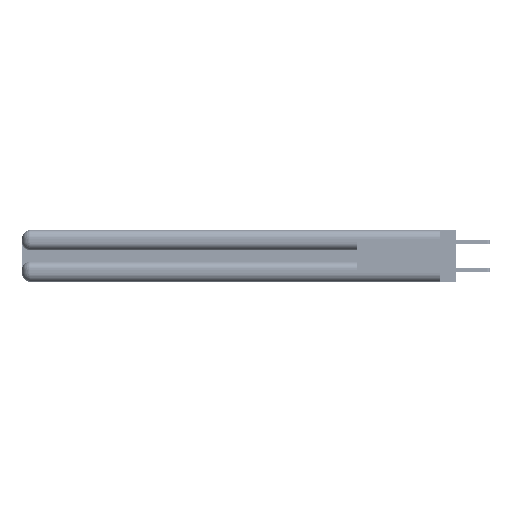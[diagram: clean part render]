
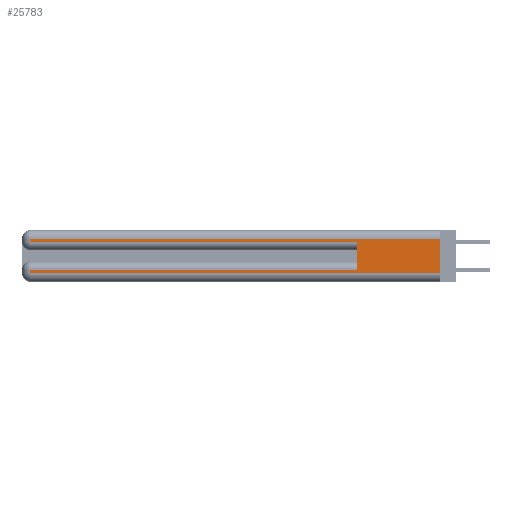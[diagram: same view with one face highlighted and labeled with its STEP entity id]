
A CAD part, left-side view. The second image highlights one B-rep face of the part: STEP entity #25783.
In plain terms, the highlighted planar face has unit normal (-1, 0, 0).
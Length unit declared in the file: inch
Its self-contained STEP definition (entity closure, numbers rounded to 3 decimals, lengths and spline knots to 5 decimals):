
#745 = EDGE_CURVE ( 'NONE', #26347, #50135, #25596, .T. ) ;
#1345 = CARTESIAN_POINT ( 'NONE',  ( 0., 0., 0.085 ) ) ;
#2168 = VERTEX_POINT ( 'NONE', #16665 ) ;
#4314 = CARTESIAN_POINT ( 'NONE',  ( 0., 2.94, 0.31 ) ) ;
#6376 = VERTEX_POINT ( 'NONE', #28918 ) ;
#7608 = PLANE ( 'NONE',  #21786 ) ;
#8194 = EDGE_CURVE ( 'NONE', #26347, #46126, #44159, .T. ) ;
#8796 = CARTESIAN_POINT ( 'NONE',  ( 0., 0.6, 0.285 ) ) ;
#9273 = ORIENTED_EDGE ( 'NONE', *, *, #20808, .T. ) ;
#9450 = ORIENTED_EDGE ( 'NONE', *, *, #745, .F. ) ;
#10535 = LINE ( 'NONE', #53746, #53653 ) ;
#10716 = LINE ( 'NONE', #10890, #23143 ) ;
#10890 = CARTESIAN_POINT ( 'NONE',  ( 0., 0., 0.285 ) ) ;
#10915 = CARTESIAN_POINT ( 'NONE',  ( 0., 0., 0.06 ) ) ;
#11662 = DIRECTION ( 'NONE',  ( 0., 0., 1. ) ) ;
#14680 = VECTOR ( 'NONE', #11662, 39.37008 ) ;
#14950 = VECTOR ( 'NONE', #29302, 39.37008 ) ;
#15764 = DIRECTION ( 'NONE',  ( 0., -1., 0. ) ) ;
#16665 = CARTESIAN_POINT ( 'NONE',  ( 0., 2.94, 0.06 ) ) ;
#16759 = EDGE_CURVE ( 'NONE', #42700, #2168, #10535, .T. ) ;
#19677 = CARTESIAN_POINT ( 'NONE',  ( 0., 2.94, 0.37 ) ) ;
#20808 = EDGE_CURVE ( 'NONE', #2168, #50135, #25682, .T. ) ;
#21786 = AXIS2_PLACEMENT_3D ( 'NONE', #25414, #38299, #34571 ) ;
#23143 = VECTOR ( 'NONE', #41982, 39.37008 ) ;
#23266 = EDGE_LOOP ( 'NONE', ( #9450, #26872, #36461, #52309, #53815, #45642, #42900, #9273 ) ) ;
#24949 = VECTOR ( 'NONE', #15764, 39.37008 ) ;
#25392 = VECTOR ( 'NONE', #55102, 39.37008 ) ;
#25414 = CARTESIAN_POINT ( 'NONE',  ( 0., 0., 0.37 ) ) ;
#25596 = LINE ( 'NONE', #37191, #54187 ) ;
#25682 = LINE ( 'NONE', #10915, #24949 ) ;
#25783 = ADVANCED_FACE ( 'NONE', ( #51141 ), #7608, .F. ) ;
#26238 = EDGE_CURVE ( 'NONE', #49688, #30802, #10716, .T. ) ;
#26347 = VERTEX_POINT ( 'NONE', #55228 ) ;
#26872 = ORIENTED_EDGE ( 'NONE', *, *, #8194, .T. ) ;
#28918 = CARTESIAN_POINT ( 'NONE',  ( 0., 0.6, 0.085 ) ) ;
#29302 = DIRECTION ( 'NONE',  ( 0., 1., 0. ) ) ;
#30802 = VERTEX_POINT ( 'NONE', #8796 ) ;
#33212 = CARTESIAN_POINT ( 'NONE',  ( 0., 0., 0.31 ) ) ;
#34571 = DIRECTION ( 'NONE',  ( 0., 0., -1. ) ) ;
#35646 = EDGE_CURVE ( 'NONE', #6376, #30802, #49414, .T. ) ;
#36461 = ORIENTED_EDGE ( 'NONE', *, *, #36992, .T. ) ;
#36992 = EDGE_CURVE ( 'NONE', #46126, #49688, #57228, .T. ) ;
#37191 = CARTESIAN_POINT ( 'NONE',  ( 0., 0., 0.37 ) ) ;
#38299 = DIRECTION ( 'NONE',  ( 1., 0., 0. ) ) ;
#41982 = DIRECTION ( 'NONE',  ( 0., -1., 0. ) ) ;
#42560 = CARTESIAN_POINT ( 'NONE',  ( 0., 0.6, 0.145 ) ) ;
#42700 = VERTEX_POINT ( 'NONE', #54254 ) ;
#42859 = LINE ( 'NONE', #1345, #25392 ) ;
#42900 = ORIENTED_EDGE ( 'NONE', *, *, #16759, .T. ) ;
#44159 = LINE ( 'NONE', #33212, #14950 ) ;
#44593 = DIRECTION ( 'NONE',  ( 0., 0., -1. ) ) ;
#45642 = ORIENTED_EDGE ( 'NONE', *, *, #54660, .T. ) ;
#46126 = VERTEX_POINT ( 'NONE', #4314 ) ;
#46189 = DIRECTION ( 'NONE',  ( 0., 0., -1. ) ) ;
#46527 = DIRECTION ( 'NONE',  ( 0., 0., -1. ) ) ;
#49414 = LINE ( 'NONE', #42560, #14680 ) ;
#49564 = VECTOR ( 'NONE', #46527, 39.37008 ) ;
#49688 = VERTEX_POINT ( 'NONE', #57032 ) ;
#50135 = VERTEX_POINT ( 'NONE', #51730 ) ;
#51141 = FACE_OUTER_BOUND ( 'NONE', #23266, .T. ) ;
#51730 = CARTESIAN_POINT ( 'NONE',  ( 0., 0., 0.06 ) ) ;
#52309 = ORIENTED_EDGE ( 'NONE', *, *, #26238, .T. ) ;
#53653 = VECTOR ( 'NONE', #44593, 39.37008 ) ;
#53746 = CARTESIAN_POINT ( 'NONE',  ( 0., 2.94, 0.37 ) ) ;
#53815 = ORIENTED_EDGE ( 'NONE', *, *, #35646, .F. ) ;
#54187 = VECTOR ( 'NONE', #46189, 39.37008 ) ;
#54254 = CARTESIAN_POINT ( 'NONE',  ( 0., 2.94, 0.085 ) ) ;
#54660 = EDGE_CURVE ( 'NONE', #6376, #42700, #42859, .T. ) ;
#55102 = DIRECTION ( 'NONE',  ( 0., 1., 0. ) ) ;
#55228 = CARTESIAN_POINT ( 'NONE',  ( 0., 0., 0.31 ) ) ;
#57032 = CARTESIAN_POINT ( 'NONE',  ( 0., 2.94, 0.285 ) ) ;
#57228 = LINE ( 'NONE', #19677, #49564 ) ;
